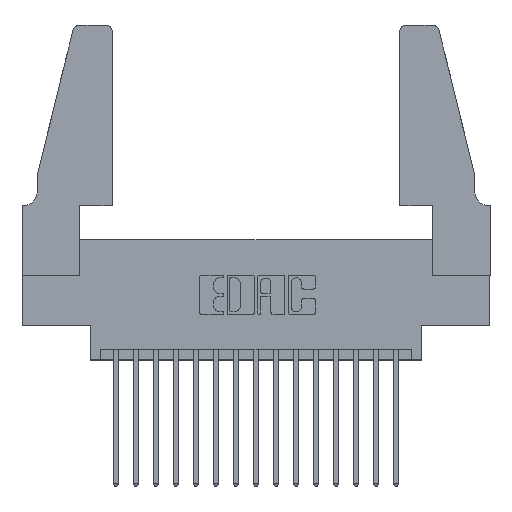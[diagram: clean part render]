
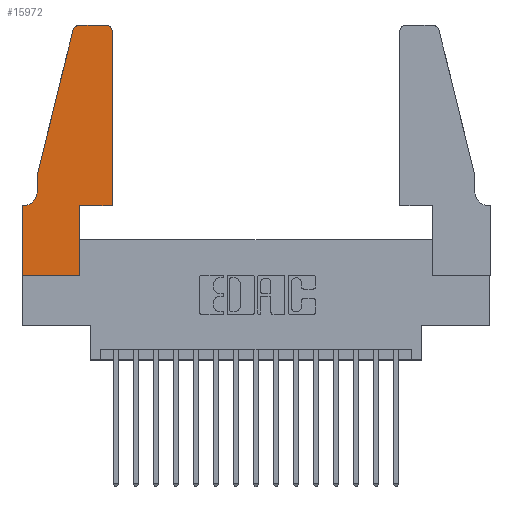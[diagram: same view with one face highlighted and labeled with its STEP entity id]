
A CAD part, top view. The second image highlights one B-rep face of the part: STEP entity #15972.
In plain terms, the highlighted planar face has unit normal (0, 0, 1).
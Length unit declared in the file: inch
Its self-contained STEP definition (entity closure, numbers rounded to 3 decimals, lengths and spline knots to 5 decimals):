
#139 = LINE ( 'NONE', #7005, #3387 ) ;
#392 = CARTESIAN_POINT ( 'NONE',  ( 0.4505, 0.35, 0.37 ) ) ;
#572 = EDGE_CURVE ( 'NONE', #16234, #9522, #13088, .T. ) ;
#597 = EDGE_CURVE ( 'NONE', #1396, #11092, #6881, .T. ) ;
#705 = DIRECTION ( 'NONE',  ( 0., 0., 1. ) ) ;
#739 = DIRECTION ( 'NONE',  ( 1., 0., 0. ) ) ;
#802 = AXIS2_PLACEMENT_3D ( 'NONE', #7425, #14253, #739 ) ;
#866 = DIRECTION ( 'NONE',  ( 0., 1., 0. ) ) ;
#1287 = ORIENTED_EDGE ( 'NONE', *, *, #13260, .T. ) ;
#1396 = VERTEX_POINT ( 'NONE', #2951 ) ;
#1638 = EDGE_CURVE ( 'NONE', #11092, #14310, #1976, .T. ) ;
#1744 = CARTESIAN_POINT ( 'NONE',  ( 0.4505, 1.22, 0.37 ) ) ;
#1879 = CARTESIAN_POINT ( 'NONE',  ( 0., 0., 0.37 ) ) ;
#1976 = LINE ( 'NONE', #6202, #5807 ) ;
#1990 = CARTESIAN_POINT ( 'NONE',  ( 0.0755, 0.35, 0.37 ) ) ;
#2429 = VECTOR ( 'NONE', #5401, 39.37008 ) ;
#2670 = VERTEX_POINT ( 'NONE', #6005 ) ;
#2846 = LINE ( 'NONE', #3319, #9667 ) ;
#2946 = DIRECTION ( 'NONE',  ( -1., 0., 0. ) ) ;
#2951 = CARTESIAN_POINT ( 'NONE',  ( 0.2865, 0.35, 0.37 ) ) ;
#3207 = VERTEX_POINT ( 'NONE', #10006 ) ;
#3273 = LINE ( 'NONE', #16712, #2429 ) ;
#3319 = CARTESIAN_POINT ( 'NONE',  ( 0.2605, 1.25, 0.37 ) ) ;
#3376 = DIRECTION ( 'NONE',  ( 1., 0., 0. ) ) ;
#3387 = VECTOR ( 'NONE', #5610, 39.37008 ) ;
#3533 = ORIENTED_EDGE ( 'NONE', *, *, #7470, .T. ) ;
#4052 = CARTESIAN_POINT ( 'NONE',  ( 0.2865, 0., 0.37 ) ) ;
#4190 = EDGE_CURVE ( 'NONE', #3207, #6553, #8391, .T. ) ;
#4596 = CARTESIAN_POINT ( 'NONE',  ( 0.0755, 0.5, 0.37 ) ) ;
#4728 = VECTOR ( 'NONE', #16900, 39.37008 ) ;
#4985 = VECTOR ( 'NONE', #15568, 39.37008 ) ;
#5195 = CIRCLE ( 'NONE', #10886, 0.03 ) ;
#5401 = DIRECTION ( 'NONE',  ( 0., 1., 0. ) ) ;
#5607 = CARTESIAN_POINT ( 'NONE',  ( 0.25487, 1.22718, 0.37 ) ) ;
#5610 = DIRECTION ( 'NONE',  ( -0.239, -0.971, 0. ) ) ;
#5637 = ORIENTED_EDGE ( 'NONE', *, *, #4190, .T. ) ;
#5807 = VECTOR ( 'NONE', #866, 39.37008 ) ;
#6005 = CARTESIAN_POINT ( 'NONE',  ( 0.0755, 0.5, 0.37 ) ) ;
#6076 = ORIENTED_EDGE ( 'NONE', *, *, #14930, .T. ) ;
#6166 = VECTOR ( 'NONE', #7438, 39.37008 ) ;
#6202 = CARTESIAN_POINT ( 'NONE',  ( 0.4505, 0.35, 0.37 ) ) ;
#6379 = CARTESIAN_POINT ( 'NONE',  ( 0.4205, 1.25, 0.37 ) ) ;
#6427 = CARTESIAN_POINT ( 'NONE',  ( 0.4505, 0.35, 0.37 ) ) ;
#6553 = VERTEX_POINT ( 'NONE', #11646 ) ;
#6573 = VERTEX_POINT ( 'NONE', #6379 ) ;
#6620 = CARTESIAN_POINT ( 'NONE',  ( 0., 0., 0.37 ) ) ;
#6881 = LINE ( 'NONE', #392, #13723 ) ;
#6920 = CARTESIAN_POINT ( 'NONE',  ( 0.0055, 0.42, 0.37 ) ) ;
#6934 = EDGE_CURVE ( 'NONE', #2670, #11675, #17064, .T. ) ;
#7005 = CARTESIAN_POINT ( 'NONE',  ( 0.0755, 0.5, 0.37 ) ) ;
#7073 = FACE_OUTER_BOUND ( 'NONE', #15338, .T. ) ;
#7425 = CARTESIAN_POINT ( 'NONE',  ( 0.4205, 1.22, 0.37 ) ) ;
#7438 = DIRECTION ( 'NONE',  ( 0., -1., 0. ) ) ;
#7470 = EDGE_CURVE ( 'NONE', #9652, #2670, #139, .T. ) ;
#7559 = CIRCLE ( 'NONE', #802, 0.03 ) ;
#8086 = AXIS2_PLACEMENT_3D ( 'NONE', #12919, #705, #3376 ) ;
#8251 = CARTESIAN_POINT ( 'NONE',  ( 0., 0., 0.37 ) ) ;
#8294 = LINE ( 'NONE', #6620, #15097 ) ;
#8391 = LINE ( 'NONE', #1990, #4985 ) ;
#8797 = EDGE_CURVE ( 'NONE', #11168, #9652, #5195, .T. ) ;
#9443 = DIRECTION ( 'NONE',  ( 0., -1., 0. ) ) ;
#9522 = VERTEX_POINT ( 'NONE', #4052 ) ;
#9652 = VERTEX_POINT ( 'NONE', #5607 ) ;
#9667 = VECTOR ( 'NONE', #15475, 39.37008 ) ;
#9887 = DIRECTION ( 'NONE',  ( 1., 0., 0. ) ) ;
#10002 = ORIENTED_EDGE ( 'NONE', *, *, #6934, .T. ) ;
#10006 = CARTESIAN_POINT ( 'NONE',  ( 0.0055, 0.35, 0.37 ) ) ;
#10327 = CIRCLE ( 'NONE', #14698, 0.07 ) ;
#10783 = ORIENTED_EDGE ( 'NONE', *, *, #15489, .T. ) ;
#10886 = AXIS2_PLACEMENT_3D ( 'NONE', #16181, #17387, #17327 ) ;
#11092 = VERTEX_POINT ( 'NONE', #6427 ) ;
#11101 = ORIENTED_EDGE ( 'NONE', *, *, #11443, .T. ) ;
#11168 = VERTEX_POINT ( 'NONE', #13243 ) ;
#11443 = EDGE_CURVE ( 'NONE', #6553, #16234, #8294, .T. ) ;
#11646 = CARTESIAN_POINT ( 'NONE',  ( 0., 0.35, 0.37 ) ) ;
#11675 = VERTEX_POINT ( 'NONE', #15995 ) ;
#12919 = CARTESIAN_POINT ( 'NONE',  ( 0., 0.35, 0.37 ) ) ;
#13088 = LINE ( 'NONE', #1879, #4728 ) ;
#13243 = CARTESIAN_POINT ( 'NONE',  ( 0.284, 1.25, 0.37 ) ) ;
#13260 = EDGE_CURVE ( 'NONE', #14310, #6573, #7559, .T. ) ;
#13723 = VECTOR ( 'NONE', #9887, 39.37008 ) ;
#13910 = DIRECTION ( 'NONE',  ( 0., 0., -1. ) ) ;
#14253 = DIRECTION ( 'NONE',  ( 0., 0., 1. ) ) ;
#14310 = VERTEX_POINT ( 'NONE', #1744 ) ;
#14698 = AXIS2_PLACEMENT_3D ( 'NONE', #6920, #13910, #2946 ) ;
#14930 = EDGE_CURVE ( 'NONE', #9522, #1396, #3273, .T. ) ;
#15097 = VECTOR ( 'NONE', #9443, 39.37008 ) ;
#15338 = EDGE_LOOP ( 'NONE', ( #16146, #16785, #3533, #10002, #10783, #5637, #11101, #16332, #6076, #16577, #17302, #1287 ) ) ;
#15475 = DIRECTION ( 'NONE',  ( -1., 0., 0. ) ) ;
#15489 = EDGE_CURVE ( 'NONE', #11675, #3207, #10327, .T. ) ;
#15568 = DIRECTION ( 'NONE',  ( -1., 0., 0. ) ) ;
#15883 = EDGE_CURVE ( 'NONE', #6573, #11168, #2846, .T. ) ;
#15972 = ADVANCED_FACE ( 'NONE', ( #7073 ), #17217, .T. ) ;
#15995 = CARTESIAN_POINT ( 'NONE',  ( 0.0755, 0.42, 0.37 ) ) ;
#16146 = ORIENTED_EDGE ( 'NONE', *, *, #15883, .T. ) ;
#16181 = CARTESIAN_POINT ( 'NONE',  ( 0.284, 1.22, 0.37 ) ) ;
#16234 = VERTEX_POINT ( 'NONE', #8251 ) ;
#16332 = ORIENTED_EDGE ( 'NONE', *, *, #572, .T. ) ;
#16577 = ORIENTED_EDGE ( 'NONE', *, *, #597, .T. ) ;
#16712 = CARTESIAN_POINT ( 'NONE',  ( 0.2865, 0.35, 0.37 ) ) ;
#16785 = ORIENTED_EDGE ( 'NONE', *, *, #8797, .T. ) ;
#16900 = DIRECTION ( 'NONE',  ( 1., 0., 0. ) ) ;
#17064 = LINE ( 'NONE', #4596, #6166 ) ;
#17217 = PLANE ( 'NONE',  #8086 ) ;
#17302 = ORIENTED_EDGE ( 'NONE', *, *, #1638, .T. ) ;
#17327 = DIRECTION ( 'NONE',  ( 1., 0., 0. ) ) ;
#17387 = DIRECTION ( 'NONE',  ( 0., 0., 1. ) ) ;
